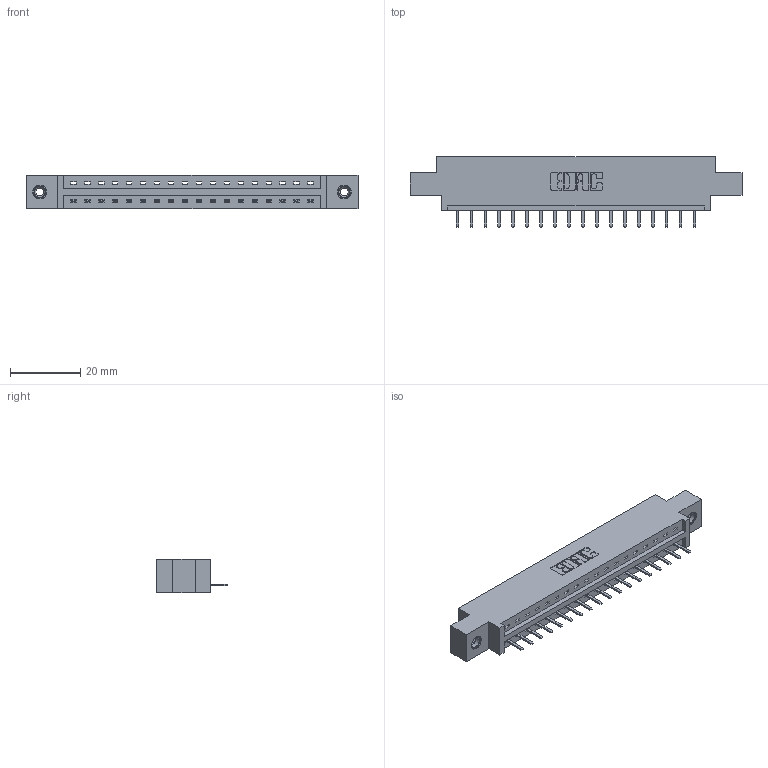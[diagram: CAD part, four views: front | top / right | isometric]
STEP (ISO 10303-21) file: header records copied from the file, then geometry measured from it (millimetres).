
FILE_DESCRIPTION (( 'STEP AP203' ), '1' );
FILE_NAME ('387-018-520-608.STEP', '2019-10-02T19:51:26', ( '' ), ( '' ), 'SwSTEP 2.0', 'SolidWorks 2016', '' );
FILE_SCHEMA (( 'CONFIG_CONTROL_DESIGN' ));
Length unit declared in the file: inch
Products named in the file (4): 387-018-520-608; 345-250-001_345-250-003-102; 345-292-001_345-293-120; 337 Part_0.170 Offset - 0.156 Dia-TI
Assembly tree (21 placements, depth 2):
  387-018-520-608
    337 Part_0.170 Offset - 0.156 Dia-TI
    345-292-001_345-293-120  x18
    345-250-001_345-250-003-102  x2
Bounding box: 94.34 x 20.02 x 9.4 mm (x, y, z)
Volume: 9328.5 mm3; surface area: 9446.1 mm2
Topology: 21 solids, 21 shells, 1366 faces, 3987 edges, 2602 vertices
Faces by surface type: plane 970, cylinder 380, cone 12, torus 4
Entity records: 17916 total; most frequent: CARTESIAN_POINT 3111, ORIENTED_EDGE 3046, DIRECTION 2689, EDGE_CURVE 1523, LINE 1371, VECTOR 1371, VERTEX_POINT 1008, AXIS2_PLACEMENT_3D 659
